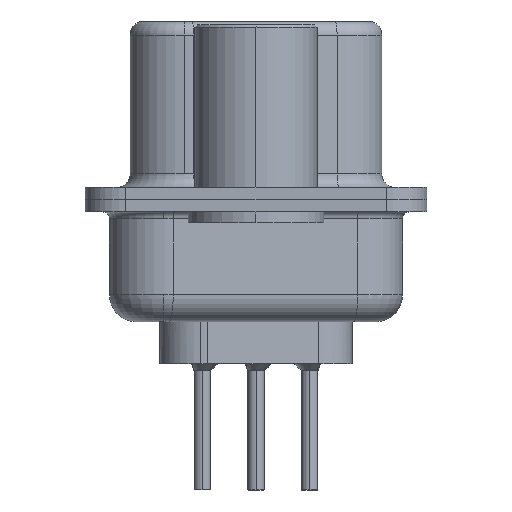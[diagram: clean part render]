
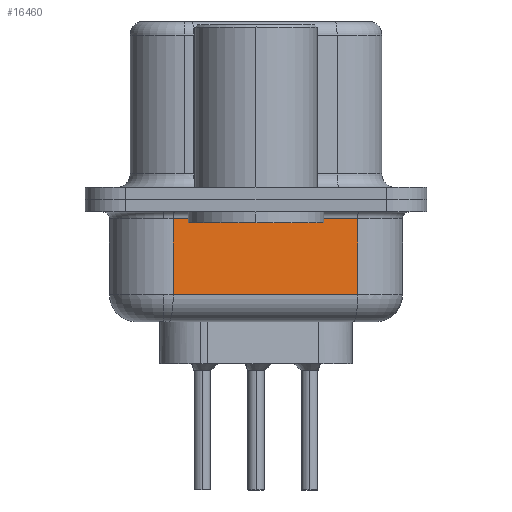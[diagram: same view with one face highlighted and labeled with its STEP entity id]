
A CAD part, left-side view. The second image highlights one B-rep face of the part: STEP entity #16460.
In plain terms, the highlighted planar face has unit normal (-0.985, -0.174, 0).
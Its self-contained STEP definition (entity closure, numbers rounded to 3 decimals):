
#399 = ORIENTED_EDGE ( 'NONE', *, *, #22658, .F. ) ;
#645 = DIRECTION ( 'NONE',  ( -0.174, 0.985, 0. ) ) ;
#1546 = EDGE_CURVE ( 'NONE', #20913, #7031, #19153, .T. ) ;
#3160 = CARTESIAN_POINT ( 'NONE',  ( 2.925, 3.053, -0.7 ) ) ;
#4305 = PLANE ( 'NONE',  #16042 ) ;
#4345 = CARTESIAN_POINT ( 'NONE',  ( 2.925, 3.053, -0.7 ) ) ;
#6374 = DIRECTION ( 'NONE',  ( 0.174, -0.985, 0. ) ) ;
#6744 = VECTOR ( 'NONE', #21243, 1000. ) ;
#6839 = EDGE_CURVE ( 'NONE', #7031, #9038, #22696, .T. ) ;
#7031 = VERTEX_POINT ( 'NONE', #19762 ) ;
#7765 = ORIENTED_EDGE ( 'NONE', *, *, #12161, .T. ) ;
#9038 = VERTEX_POINT ( 'NONE', #3160 ) ;
#10214 = VECTOR ( 'NONE', #11820, 1000. ) ;
#10814 = CARTESIAN_POINT ( 'NONE',  ( 4.124, -3.747, -3.5 ) ) ;
#11056 = CARTESIAN_POINT ( 'NONE',  ( 2.925, 3.053, -3.5 ) ) ;
#11820 = DIRECTION ( 'NONE',  ( -0.174, 0.985, 0. ) ) ;
#12161 = EDGE_CURVE ( 'NONE', #16294, #20913, #15811, .T. ) ;
#14769 = VECTOR ( 'NONE', #6374, 1000. ) ;
#15211 = FACE_OUTER_BOUND ( 'NONE', #22593, .T. ) ;
#15811 = LINE ( 'NONE', #23257, #14769 ) ;
#16042 = AXIS2_PLACEMENT_3D ( 'NONE', #20717, #17422, #645 ) ;
#16294 = VERTEX_POINT ( 'NONE', #11056 ) ;
#16460 = ADVANCED_FACE ( 'NONE', ( #15211 ), #4305, .F. ) ;
#17085 = CARTESIAN_POINT ( 'NONE',  ( 4.124, -3.747, -4.5 ) ) ;
#17246 = VECTOR ( 'NONE', #23589, 1000. ) ;
#17422 = DIRECTION ( 'NONE',  ( 0.985, 0.174, 0. ) ) ;
#18332 = LINE ( 'NONE', #19913, #17246 ) ;
#19153 = LINE ( 'NONE', #17085, #6744 ) ;
#19762 = CARTESIAN_POINT ( 'NONE',  ( 4.124, -3.747, -0.7 ) ) ;
#19913 = CARTESIAN_POINT ( 'NONE',  ( 2.925, 3.053, -4.5 ) ) ;
#20717 = CARTESIAN_POINT ( 'NONE',  ( 2.925, 3.053, -4.5 ) ) ;
#20913 = VERTEX_POINT ( 'NONE', #10814 ) ;
#21243 = DIRECTION ( 'NONE',  ( 0., 0., 1. ) ) ;
#21380 = ORIENTED_EDGE ( 'NONE', *, *, #6839, .T. ) ;
#22593 = EDGE_LOOP ( 'NONE', ( #399, #7765, #23254, #21380 ) ) ;
#22658 = EDGE_CURVE ( 'NONE', #16294, #9038, #18332, .T. ) ;
#22696 = LINE ( 'NONE', #4345, #10214 ) ;
#23254 = ORIENTED_EDGE ( 'NONE', *, *, #1546, .T. ) ;
#23257 = CARTESIAN_POINT ( 'NONE',  ( 2.925, 3.053, -3.5 ) ) ;
#23589 = DIRECTION ( 'NONE',  ( 0., 0., 1. ) ) ;
